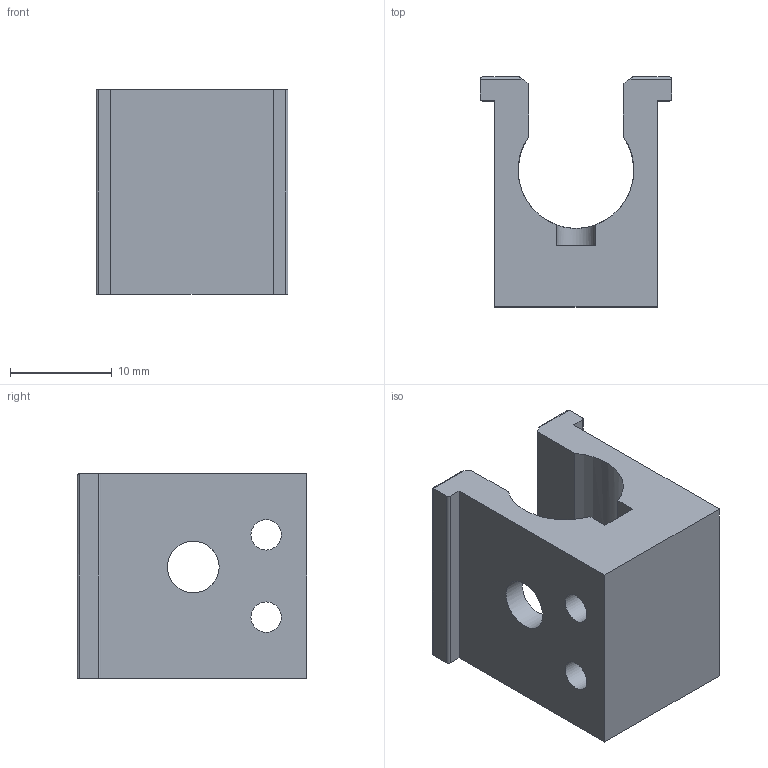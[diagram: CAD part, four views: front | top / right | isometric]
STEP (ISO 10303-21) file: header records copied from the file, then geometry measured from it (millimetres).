
FILE_DESCRIPTION(/* description */ ('RECEIVER'),/* implementation_level */ '2;1');
FILE_NAME(/* name */ '3011 Front Rail.stp',/* time_stamp */ '2021-05-11T13:26:48-05:00',/* author */ ('johne'),/* organization */ (''),/* preprocessor_version */ 'ST-DEVELOPER v18',/* originating_system */ 'Autodesk Inventor 2020',/* authorisation */ '');
FILE_SCHEMA (('AUTOMOTIVE_DESIGN { 1 0 10303 214 3 1 1 }'));
Length unit declared in the file: inch
Products named in the file (1): 3011 front rail
Bounding box: 18.88 x 22.61 x 20.12 mm (x, y, z)
Volume: 4094.1 mm3; surface area: 2989 mm2
Topology: 1 solids, 1 shells, 30 faces, 86 edges, 58 vertices
Faces by surface type: plane 16, cylinder 14
Full cylindrical faces by diameter (mm): 3 x2, 5.105 x2
Entity records: 1161 total; most frequent: CARTESIAN_POINT 292, ORIENTED_EDGE 172, DIRECTION 165, EDGE_CURVE 86, VERTEX_POINT 58, LINE 55, VECTOR 55, AXIS2_PLACEMENT_3D 55
